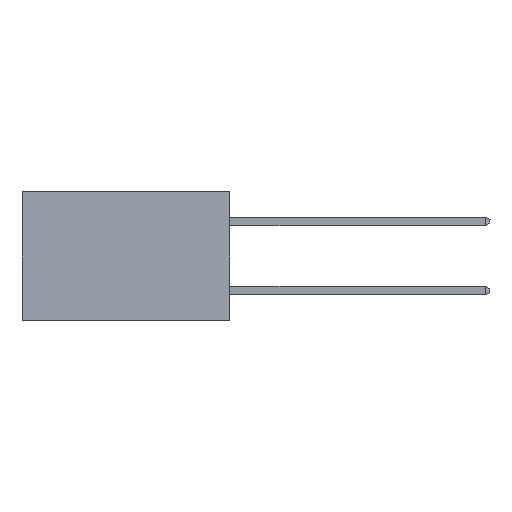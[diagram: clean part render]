
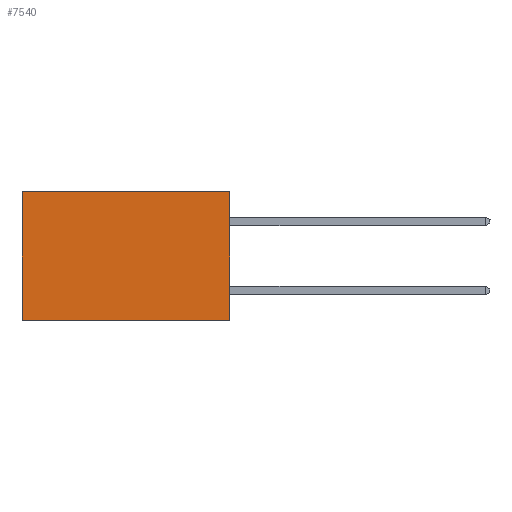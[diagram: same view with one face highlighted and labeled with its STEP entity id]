
A CAD part, left-side view. The second image highlights one B-rep face of the part: STEP entity #7540.
In plain terms, the highlighted planar face has unit normal (-1, 0, 0).
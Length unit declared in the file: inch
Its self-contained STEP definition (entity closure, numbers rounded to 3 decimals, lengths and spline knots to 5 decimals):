
#1008 = LINE ( 'NONE', #5369, #7809 ) ;
#1278 = DIRECTION ( 'NONE',  ( 0., 1., 0. ) ) ;
#1369 = LINE ( 'NONE', #8727, #9296 ) ;
#1553 = ORIENTED_EDGE ( 'NONE', *, *, #11386, .T. ) ;
#1631 = DIRECTION ( 'NONE',  ( 0., 0., -1. ) ) ;
#2847 = EDGE_CURVE ( 'NONE', #6763, #18491, #16998, .T. ) ;
#3976 = DIRECTION ( 'NONE',  ( 0., 0., -1. ) ) ;
#4283 = VERTEX_POINT ( 'NONE', #12971 ) ;
#5343 = LINE ( 'NONE', #13021, #7367 ) ;
#5369 = CARTESIAN_POINT ( 'NONE',  ( 0.2615, 0., 0. ) ) ;
#6763 = VERTEX_POINT ( 'NONE', #12165 ) ;
#6928 = DIRECTION ( 'NONE',  ( 0., 1., 0. ) ) ;
#7367 = VECTOR ( 'NONE', #1631, 39.37008 ) ;
#7540 = ADVANCED_FACE ( 'NONE', ( #16285 ), #10419, .F. ) ;
#7552 = DIRECTION ( 'NONE',  ( 0., 0., -1. ) ) ;
#7809 = VECTOR ( 'NONE', #6928, 39.37008 ) ;
#8727 = CARTESIAN_POINT ( 'NONE',  ( 0.2615, 0., -0.37 ) ) ;
#8990 = CARTESIAN_POINT ( 'NONE',  ( 0.2615, 0., -0.37 ) ) ;
#9021 = CARTESIAN_POINT ( 'NONE',  ( 0.2615, 0., -0.37 ) ) ;
#9296 = VECTOR ( 'NONE', #1278, 39.37008 ) ;
#10223 = EDGE_CURVE ( 'NONE', #18491, #4283, #1369, .T. ) ;
#10419 = PLANE ( 'NONE',  #14859 ) ;
#11239 = CARTESIAN_POINT ( 'NONE',  ( 0.2615, 0., -0.37 ) ) ;
#11386 = EDGE_CURVE ( 'NONE', #6763, #17999, #1008, .T. ) ;
#12086 = ORIENTED_EDGE ( 'NONE', *, *, #18776, .T. ) ;
#12165 = CARTESIAN_POINT ( 'NONE',  ( 0.2615, 0., 0. ) ) ;
#12971 = CARTESIAN_POINT ( 'NONE',  ( 0.2615, 0.6, -0.37 ) ) ;
#13021 = CARTESIAN_POINT ( 'NONE',  ( 0.2615, 0.6, -0.37 ) ) ;
#14013 = ORIENTED_EDGE ( 'NONE', *, *, #2847, .F. ) ;
#14839 = DIRECTION ( 'NONE',  ( 1., 0., 0. ) ) ;
#14859 = AXIS2_PLACEMENT_3D ( 'NONE', #8990, #14839, #7552 ) ;
#15288 = EDGE_LOOP ( 'NONE', ( #12086, #16097, #14013, #1553 ) ) ;
#16097 = ORIENTED_EDGE ( 'NONE', *, *, #10223, .F. ) ;
#16285 = FACE_OUTER_BOUND ( 'NONE', #15288, .T. ) ;
#16998 = LINE ( 'NONE', #11239, #18314 ) ;
#17478 = CARTESIAN_POINT ( 'NONE',  ( 0.2615, 0.6, 0. ) ) ;
#17999 = VERTEX_POINT ( 'NONE', #17478 ) ;
#18314 = VECTOR ( 'NONE', #3976, 39.37008 ) ;
#18491 = VERTEX_POINT ( 'NONE', #9021 ) ;
#18776 = EDGE_CURVE ( 'NONE', #17999, #4283, #5343, .T. ) ;
